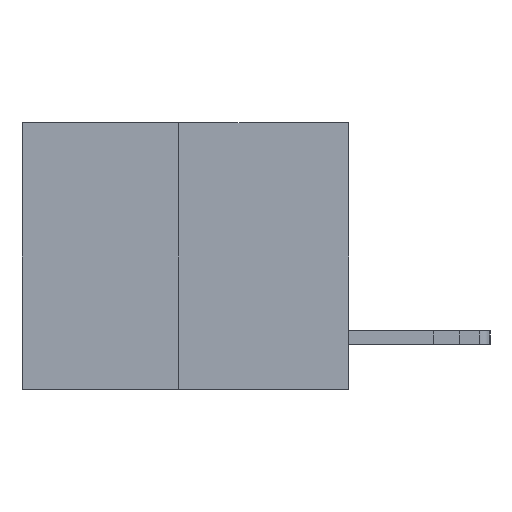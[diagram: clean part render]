
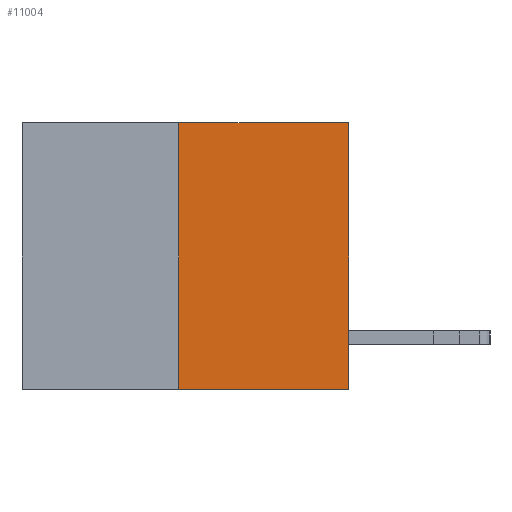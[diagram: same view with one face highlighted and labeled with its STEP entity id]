
A CAD part, left-side view. The second image highlights one B-rep face of the part: STEP entity #11004.
In plain terms, the highlighted planar face has unit normal (-1, 0, 0).
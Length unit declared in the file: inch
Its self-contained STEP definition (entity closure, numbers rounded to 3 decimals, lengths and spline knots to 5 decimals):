
#84 = EDGE_LOOP ( 'NONE', ( #12572, #15423, #18821, #4100 ) ) ;
#291 = DIRECTION ( 'NONE',  ( 1., 0., 0. ) ) ;
#605 = DIRECTION ( 'NONE',  ( 0., 0., 1. ) ) ;
#1765 = VECTOR ( 'NONE', #605, 39.37008 ) ;
#2250 = EDGE_CURVE ( 'NONE', #7683, #5286, #2756, .T. ) ;
#2739 = AXIS2_PLACEMENT_3D ( 'NONE', #8241, #291, #11515 ) ;
#2756 = LINE ( 'NONE', #12061, #10721 ) ;
#3909 = CARTESIAN_POINT ( 'NONE',  ( 0., 0., -0.49 ) ) ;
#4100 = ORIENTED_EDGE ( 'NONE', *, *, #20073, .F. ) ;
#4899 = EDGE_CURVE ( 'NONE', #5232, #7683, #4981, .T. ) ;
#4981 = LINE ( 'NONE', #9884, #12903 ) ;
#5145 = CARTESIAN_POINT ( 'NONE',  ( 0., 0.312, -0.49 ) ) ;
#5232 = VERTEX_POINT ( 'NONE', #5145 ) ;
#5286 = VERTEX_POINT ( 'NONE', #14363 ) ;
#5466 = FACE_OUTER_BOUND ( 'NONE', #84, .T. ) ;
#5976 = EDGE_CURVE ( 'NONE', #5232, #19136, #6940, .T. ) ;
#6940 = LINE ( 'NONE', #14925, #1765 ) ;
#7683 = VERTEX_POINT ( 'NONE', #3909 ) ;
#7878 = CARTESIAN_POINT ( 'NONE',  ( 0., 0.6, 0. ) ) ;
#7943 = DIRECTION ( 'NONE',  ( 0., -1., 0. ) ) ;
#8241 = CARTESIAN_POINT ( 'NONE',  ( 0., 0.6, 0. ) ) ;
#9884 = CARTESIAN_POINT ( 'NONE',  ( 0., 0.6, -0.49 ) ) ;
#10721 = VECTOR ( 'NONE', #20025, 39.37008 ) ;
#11004 = ADVANCED_FACE ( 'NONE', ( #5466 ), #17810, .F. ) ;
#11515 = DIRECTION ( 'NONE',  ( 0., 0., -1. ) ) ;
#12061 = CARTESIAN_POINT ( 'NONE',  ( 0., 0., 0. ) ) ;
#12572 = ORIENTED_EDGE ( 'NONE', *, *, #5976, .F. ) ;
#12854 = LINE ( 'NONE', #7878, #17812 ) ;
#12903 = VECTOR ( 'NONE', #19627, 39.37008 ) ;
#14363 = CARTESIAN_POINT ( 'NONE',  ( 0., 0., 0. ) ) ;
#14925 = CARTESIAN_POINT ( 'NONE',  ( 0., 0.312, -0.49 ) ) ;
#15423 = ORIENTED_EDGE ( 'NONE', *, *, #4899, .T. ) ;
#17348 = CARTESIAN_POINT ( 'NONE',  ( 0., 0.312, 0. ) ) ;
#17810 = PLANE ( 'NONE',  #2739 ) ;
#17812 = VECTOR ( 'NONE', #7943, 39.37008 ) ;
#18821 = ORIENTED_EDGE ( 'NONE', *, *, #2250, .T. ) ;
#19136 = VERTEX_POINT ( 'NONE', #17348 ) ;
#19627 = DIRECTION ( 'NONE',  ( 0., -1., 0. ) ) ;
#20025 = DIRECTION ( 'NONE',  ( 0., 0., 1. ) ) ;
#20073 = EDGE_CURVE ( 'NONE', #19136, #5286, #12854, .T. ) ;
